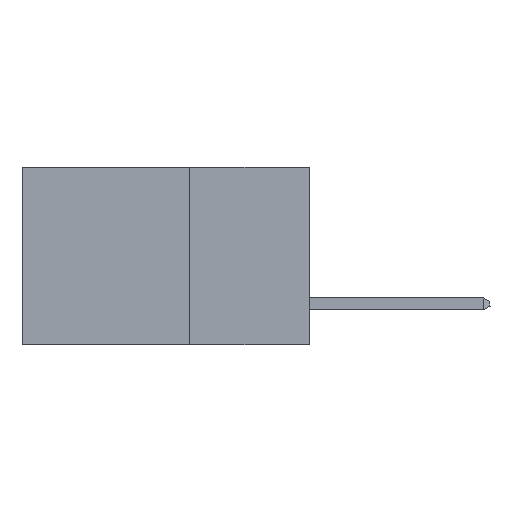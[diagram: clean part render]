
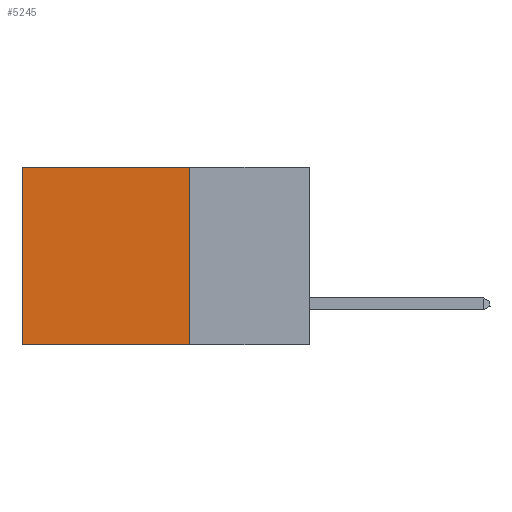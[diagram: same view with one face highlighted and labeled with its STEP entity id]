
A CAD part, left-side view. The second image highlights one B-rep face of the part: STEP entity #5245.
In plain terms, the highlighted planar face has unit normal (-1, 0, 0).
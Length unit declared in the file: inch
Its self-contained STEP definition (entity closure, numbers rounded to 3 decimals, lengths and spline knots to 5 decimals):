
#1208 = CARTESIAN_POINT ( 'NONE',  ( 0.2875, 0.25, 0. ) ) ;
#1447 = LINE ( 'NONE', #34980, #4277 ) ;
#3253 = ORIENTED_EDGE ( 'NONE', *, *, #29045, .F. ) ;
#3902 = VECTOR ( 'NONE', #8232, 39.37008 ) ;
#4277 = VECTOR ( 'NONE', #20097, 39.37008 ) ;
#4998 = CARTESIAN_POINT ( 'NONE',  ( 0.2875, 0.25, -0.37 ) ) ;
#5245 = ADVANCED_FACE ( 'NONE', ( #23534 ), #22206, .F. ) ;
#6457 = ORIENTED_EDGE ( 'NONE', *, *, #7684, .T. ) ;
#6695 = LINE ( 'NONE', #24242, #11838 ) ;
#7364 = CARTESIAN_POINT ( 'NONE',  ( 0.2875, 0.25, 0. ) ) ;
#7684 = EDGE_CURVE ( 'NONE', #29514, #30820, #1447, .T. ) ;
#8232 = DIRECTION ( 'NONE',  ( 0., 0., -1. ) ) ;
#10586 = CARTESIAN_POINT ( 'NONE',  ( 0.2875, 0.25, 0. ) ) ;
#11335 = DIRECTION ( 'NONE',  ( 0., 1., 0. ) ) ;
#11838 = VECTOR ( 'NONE', #18346, 39.37008 ) ;
#14040 = VECTOR ( 'NONE', #11335, 39.37008 ) ;
#16115 = EDGE_CURVE ( 'NONE', #38647, #18089, #33282, .T. ) ;
#17316 = EDGE_CURVE ( 'NONE', #38647, #29514, #23323, .T. ) ;
#18089 = VERTEX_POINT ( 'NONE', #4998 ) ;
#18346 = DIRECTION ( 'NONE',  ( 0., 1., 0. ) ) ;
#20097 = DIRECTION ( 'NONE',  ( 0., 0., -1. ) ) ;
#21536 = CARTESIAN_POINT ( 'NONE',  ( 0.2875, 0.6, 0. ) ) ;
#22206 = PLANE ( 'NONE',  #43358 ) ;
#23323 = LINE ( 'NONE', #7364, #14040 ) ;
#23534 = FACE_OUTER_BOUND ( 'NONE', #43340, .T. ) ;
#24242 = CARTESIAN_POINT ( 'NONE',  ( 0.2875, 0.25, -0.37 ) ) ;
#29045 = EDGE_CURVE ( 'NONE', #18089, #30820, #6695, .T. ) ;
#29514 = VERTEX_POINT ( 'NONE', #21536 ) ;
#29651 = DIRECTION ( 'NONE',  ( 0., 0., -1. ) ) ;
#29965 = DIRECTION ( 'NONE',  ( 1., 0., 0. ) ) ;
#30820 = VERTEX_POINT ( 'NONE', #40612 ) ;
#33282 = LINE ( 'NONE', #1208, #3902 ) ;
#34980 = CARTESIAN_POINT ( 'NONE',  ( 0.2875, 0.6, 0. ) ) ;
#38647 = VERTEX_POINT ( 'NONE', #10586 ) ;
#40612 = CARTESIAN_POINT ( 'NONE',  ( 0.2875, 0.6, -0.37 ) ) ;
#43340 = EDGE_LOOP ( 'NONE', ( #6457, #3253, #44138, #45671 ) ) ;
#43358 = AXIS2_PLACEMENT_3D ( 'NONE', #47686, #29965, #29651 ) ;
#44138 = ORIENTED_EDGE ( 'NONE', *, *, #16115, .F. ) ;
#45671 = ORIENTED_EDGE ( 'NONE', *, *, #17316, .T. ) ;
#47686 = CARTESIAN_POINT ( 'NONE',  ( 0.2875, 0.25, 0. ) ) ;
